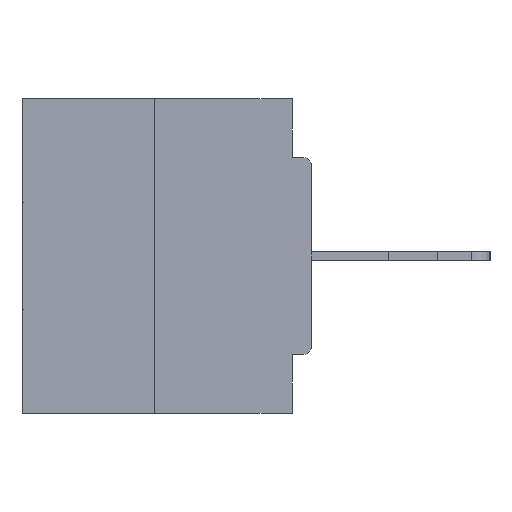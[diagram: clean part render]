
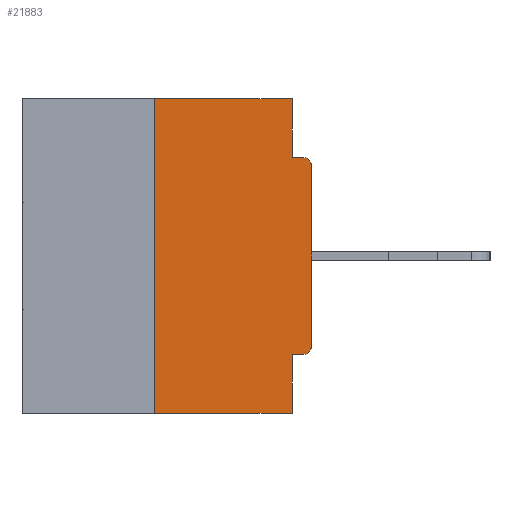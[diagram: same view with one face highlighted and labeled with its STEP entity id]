
A CAD part, left-side view. The second image highlights one B-rep face of the part: STEP entity #21883.
In plain terms, the highlighted planar face has unit normal (-1, 0, 0).
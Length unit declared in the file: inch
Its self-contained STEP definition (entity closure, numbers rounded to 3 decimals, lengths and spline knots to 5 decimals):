
#213 = DIRECTION ( 'NONE',  ( 0., -1., 0. ) ) ;
#679 = DIRECTION ( 'NONE',  ( 0., 0., 1. ) ) ;
#968 = CARTESIAN_POINT ( 'NONE',  ( 0., 0.031, -0.0935 ) ) ;
#1480 = DIRECTION ( 'NONE',  ( 0., -1., 0. ) ) ;
#1827 = EDGE_CURVE ( 'NONE', #23568, #6711, #14874, .T. ) ;
#1957 = ORIENTED_EDGE ( 'NONE', *, *, #7584, .T. ) ;
#2096 = AXIS2_PLACEMENT_3D ( 'NONE', #30099, #9365, #11779 ) ;
#2458 = CIRCLE ( 'NONE', #21178, 0.015 ) ;
#2574 = DIRECTION ( 'NONE',  ( 0., 0., -1. ) ) ;
#2805 = CARTESIAN_POINT ( 'NONE',  ( 0., 0., -0.0935 ) ) ;
#2866 = ORIENTED_EDGE ( 'NONE', *, *, #10338, .T. ) ;
#3029 = VERTEX_POINT ( 'NONE', #32222 ) ;
#4215 = DIRECTION ( 'NONE',  ( 0., 0., -1. ) ) ;
#4723 = CARTESIAN_POINT ( 'NONE',  ( 0., 0.015, -0.1085 ) ) ;
#5134 = LINE ( 'NONE', #15660, #16143 ) ;
#5882 = LINE ( 'NONE', #26454, #32658 ) ;
#6711 = VERTEX_POINT ( 'NONE', #26624 ) ;
#7555 = VERTEX_POINT ( 'NONE', #18878 ) ;
#7584 = EDGE_CURVE ( 'NONE', #12272, #15435, #2458, .T. ) ;
#7690 = EDGE_CURVE ( 'NONE', #17281, #7555, #14552, .T. ) ;
#7780 = EDGE_LOOP ( 'NONE', ( #25701, #11739, #2866, #14272, #11062, #1957, #19859, #8134, #10379, #21861 ) ) ;
#8134 = ORIENTED_EDGE ( 'NONE', *, *, #1827, .T. ) ;
#8971 = CARTESIAN_POINT ( 'NONE',  ( 0., 0., -0.3915 ) ) ;
#9206 = CARTESIAN_POINT ( 'NONE',  ( 0., 0.46, 0. ) ) ;
#9365 = DIRECTION ( 'NONE',  ( 1., 0., 0. ) ) ;
#9502 = VECTOR ( 'NONE', #679, 39.37008 ) ;
#10338 = EDGE_CURVE ( 'NONE', #25541, #25678, #32957, .T. ) ;
#10379 = ORIENTED_EDGE ( 'NONE', *, *, #22107, .F. ) ;
#10550 = DIRECTION ( 'NONE',  ( 0., 1., 0. ) ) ;
#11062 = ORIENTED_EDGE ( 'NONE', *, *, #29600, .F. ) ;
#11101 = EDGE_CURVE ( 'NONE', #15435, #23568, #14207, .T. ) ;
#11739 = ORIENTED_EDGE ( 'NONE', *, *, #13977, .F. ) ;
#11779 = DIRECTION ( 'NONE',  ( 0., 0., -1. ) ) ;
#12272 = VERTEX_POINT ( 'NONE', #29431 ) ;
#13696 = CARTESIAN_POINT ( 'NONE',  ( 0., 0., 0. ) ) ;
#13977 = EDGE_CURVE ( 'NONE', #25541, #17281, #24517, .T. ) ;
#14122 = VECTOR ( 'NONE', #29256, 39.37008 ) ;
#14201 = DIRECTION ( 'NONE',  ( -1., 0., 0. ) ) ;
#14207 = LINE ( 'NONE', #13696, #14122 ) ;
#14272 = ORIENTED_EDGE ( 'NONE', *, *, #31718, .F. ) ;
#14514 = CARTESIAN_POINT ( 'NONE',  ( 0., 0., -0.1085 ) ) ;
#14552 = LINE ( 'NONE', #9206, #18433 ) ;
#14874 = CIRCLE ( 'NONE', #28146, 0.015 ) ;
#15435 = VERTEX_POINT ( 'NONE', #8971 ) ;
#15660 = CARTESIAN_POINT ( 'NONE',  ( 0., 0.031, -0.5 ) ) ;
#16143 = VECTOR ( 'NONE', #2574, 39.37008 ) ;
#17281 = VERTEX_POINT ( 'NONE', #28607 ) ;
#18433 = VECTOR ( 'NONE', #1480, 39.37008 ) ;
#18878 = CARTESIAN_POINT ( 'NONE',  ( 0., 0.031, 0. ) ) ;
#19557 = FACE_OUTER_BOUND ( 'NONE', #7780, .T. ) ;
#19859 = ORIENTED_EDGE ( 'NONE', *, *, #11101, .T. ) ;
#21178 = AXIS2_PLACEMENT_3D ( 'NONE', #29933, #14201, #24783 ) ;
#21861 = ORIENTED_EDGE ( 'NONE', *, *, #29396, .F. ) ;
#21883 = ADVANCED_FACE ( 'NONE', ( #19557 ), #33023, .F. ) ;
#22107 = EDGE_CURVE ( 'NONE', #24811, #6711, #29207, .T. ) ;
#22192 = VECTOR ( 'NONE', #31283, 39.37008 ) ;
#23568 = VERTEX_POINT ( 'NONE', #14514 ) ;
#23815 = CARTESIAN_POINT ( 'NONE',  ( 0., 0.031, -0.5 ) ) ;
#24517 = LINE ( 'NONE', #27436, #9502 ) ;
#24783 = DIRECTION ( 'NONE',  ( 0., 0., -1. ) ) ;
#24811 = VERTEX_POINT ( 'NONE', #968 ) ;
#25541 = VERTEX_POINT ( 'NONE', #29494 ) ;
#25551 = CARTESIAN_POINT ( 'NONE',  ( 0., 0.46, -0.5 ) ) ;
#25622 = CARTESIAN_POINT ( 'NONE',  ( 0., 0.031, 0. ) ) ;
#25678 = VERTEX_POINT ( 'NONE', #23815 ) ;
#25701 = ORIENTED_EDGE ( 'NONE', *, *, #7690, .F. ) ;
#25974 = DIRECTION ( 'NONE',  ( -1., 0., 0. ) ) ;
#26454 = CARTESIAN_POINT ( 'NONE',  ( 0., 0., -0.4065 ) ) ;
#26624 = CARTESIAN_POINT ( 'NONE',  ( 0., 0.015, -0.0935 ) ) ;
#27318 = VECTOR ( 'NONE', #28308, 39.37008 ) ;
#27436 = CARTESIAN_POINT ( 'NONE',  ( 0., 0.25, 0. ) ) ;
#28146 = AXIS2_PLACEMENT_3D ( 'NONE', #4723, #25974, #4215 ) ;
#28308 = DIRECTION ( 'NONE',  ( 0., -1., 0. ) ) ;
#28607 = CARTESIAN_POINT ( 'NONE',  ( 0., 0.25, 0. ) ) ;
#29207 = LINE ( 'NONE', #2805, #31842 ) ;
#29256 = DIRECTION ( 'NONE',  ( 0., 0., 1. ) ) ;
#29396 = EDGE_CURVE ( 'NONE', #7555, #24811, #31440, .T. ) ;
#29431 = CARTESIAN_POINT ( 'NONE',  ( 0., 0.015, -0.4065 ) ) ;
#29494 = CARTESIAN_POINT ( 'NONE',  ( 0., 0.25, -0.5 ) ) ;
#29600 = EDGE_CURVE ( 'NONE', #12272, #3029, #5882, .T. ) ;
#29933 = CARTESIAN_POINT ( 'NONE',  ( 0., 0.015, -0.3915 ) ) ;
#30099 = CARTESIAN_POINT ( 'NONE',  ( 0., 0.46, 0. ) ) ;
#31283 = DIRECTION ( 'NONE',  ( 0., 0., -1. ) ) ;
#31440 = LINE ( 'NONE', #25622, #22192 ) ;
#31718 = EDGE_CURVE ( 'NONE', #3029, #25678, #5134, .T. ) ;
#31842 = VECTOR ( 'NONE', #213, 39.37008 ) ;
#32222 = CARTESIAN_POINT ( 'NONE',  ( 0., 0.031, -0.4065 ) ) ;
#32658 = VECTOR ( 'NONE', #10550, 39.37008 ) ;
#32957 = LINE ( 'NONE', #25551, #27318 ) ;
#33023 = PLANE ( 'NONE',  #2096 ) ;
